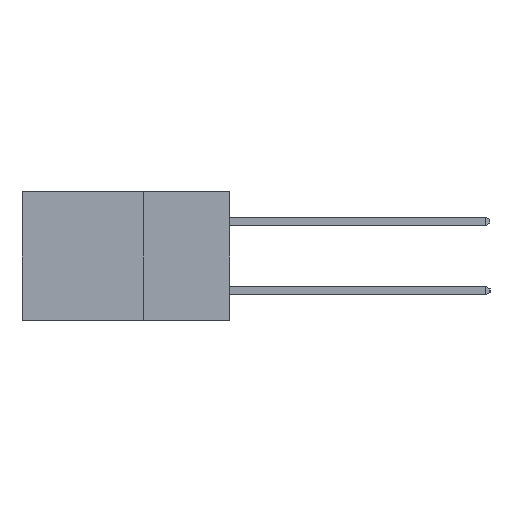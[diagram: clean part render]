
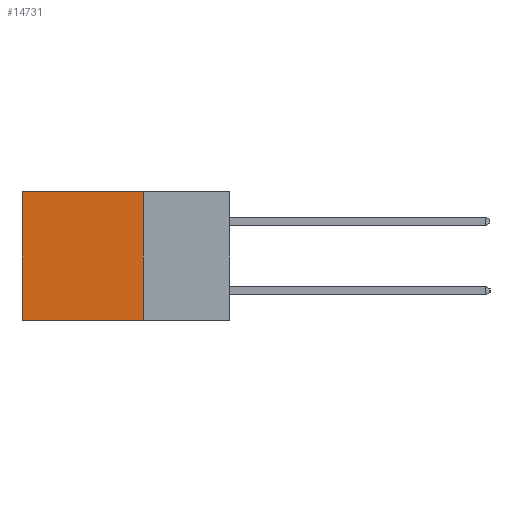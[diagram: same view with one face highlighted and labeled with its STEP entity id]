
A CAD part, left-side view. The second image highlights one B-rep face of the part: STEP entity #14731.
In plain terms, the highlighted planar face has unit normal (-1, 0, 0).
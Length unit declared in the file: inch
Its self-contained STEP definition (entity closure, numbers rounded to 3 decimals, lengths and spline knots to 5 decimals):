
#348 = VERTEX_POINT ( 'NONE', #1295 ) ;
#427 = VERTEX_POINT ( 'NONE', #5684 ) ;
#1172 = VECTOR ( 'NONE', #9391, 39.37008 ) ;
#1295 = CARTESIAN_POINT ( 'NONE',  ( 0.2615, 0.6, 0. ) ) ;
#1545 = PLANE ( 'NONE',  #5124 ) ;
#1559 = ORIENTED_EDGE ( 'NONE', *, *, #13728, .T. ) ;
#2221 = LINE ( 'NONE', #10886, #1172 ) ;
#2673 = CARTESIAN_POINT ( 'NONE',  ( 0.2615, 0.25, -0.37 ) ) ;
#2735 = CARTESIAN_POINT ( 'NONE',  ( 0.2615, 0.25, -0.37 ) ) ;
#2847 = VECTOR ( 'NONE', #10086, 39.37008 ) ;
#3024 = VERTEX_POINT ( 'NONE', #12921 ) ;
#4068 = EDGE_CURVE ( 'NONE', #3024, #6116, #13896, .T. ) ;
#4728 = CARTESIAN_POINT ( 'NONE',  ( 0.2615, 0.25, -0.37 ) ) ;
#4933 = ORIENTED_EDGE ( 'NONE', *, *, #15208, .F. ) ;
#5006 = VECTOR ( 'NONE', #10510, 39.37008 ) ;
#5124 = AXIS2_PLACEMENT_3D ( 'NONE', #4728, #6320, #16904 ) ;
#5684 = CARTESIAN_POINT ( 'NONE',  ( 0.2615, 0.6, -0.37 ) ) ;
#6116 = VERTEX_POINT ( 'NONE', #2673 ) ;
#6320 = DIRECTION ( 'NONE',  ( 1., 0., 0. ) ) ;
#7519 = LINE ( 'NONE', #8673, #2847 ) ;
#7783 = ORIENTED_EDGE ( 'NONE', *, *, #8329, .T. ) ;
#8329 = EDGE_CURVE ( 'NONE', #3024, #348, #2221, .T. ) ;
#8547 = EDGE_LOOP ( 'NONE', ( #1559, #4933, #11263, #7783 ) ) ;
#8673 = CARTESIAN_POINT ( 'NONE',  ( 0.2615, 0.6, -0.37 ) ) ;
#9391 = DIRECTION ( 'NONE',  ( 0., 1., 0. ) ) ;
#10086 = DIRECTION ( 'NONE',  ( 0., 0., -1. ) ) ;
#10375 = VECTOR ( 'NONE', #17880, 39.37008 ) ;
#10510 = DIRECTION ( 'NONE',  ( 0., 1., 0. ) ) ;
#10886 = CARTESIAN_POINT ( 'NONE',  ( 0.2615, 0.25, 0. ) ) ;
#11263 = ORIENTED_EDGE ( 'NONE', *, *, #4068, .F. ) ;
#12921 = CARTESIAN_POINT ( 'NONE',  ( 0.2615, 0.25, 0. ) ) ;
#13728 = EDGE_CURVE ( 'NONE', #348, #427, #7519, .T. ) ;
#13880 = FACE_OUTER_BOUND ( 'NONE', #8547, .T. ) ;
#13896 = LINE ( 'NONE', #17712, #10375 ) ;
#14731 = ADVANCED_FACE ( 'NONE', ( #13880 ), #1545, .F. ) ;
#15208 = EDGE_CURVE ( 'NONE', #6116, #427, #18086, .T. ) ;
#16904 = DIRECTION ( 'NONE',  ( 0., 0., -1. ) ) ;
#17712 = CARTESIAN_POINT ( 'NONE',  ( 0.2615, 0.25, -0.37 ) ) ;
#17880 = DIRECTION ( 'NONE',  ( 0., 0., -1. ) ) ;
#18086 = LINE ( 'NONE', #2735, #5006 ) ;
